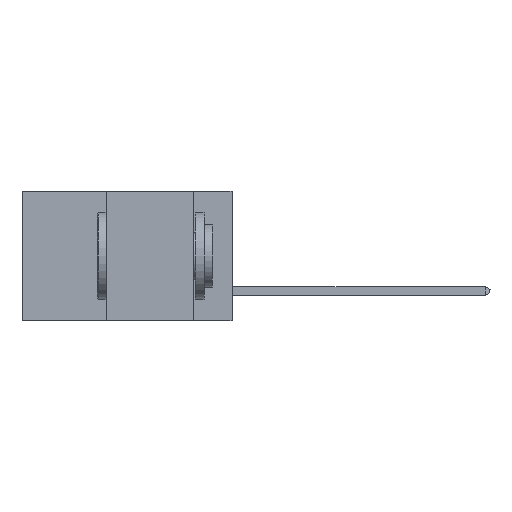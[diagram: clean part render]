
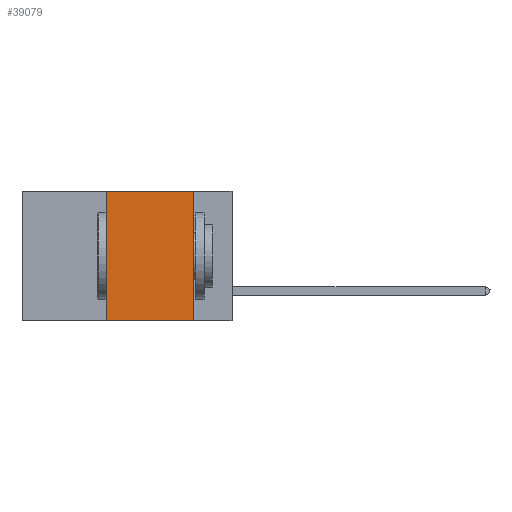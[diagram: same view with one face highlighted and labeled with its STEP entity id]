
A CAD part, left-side view. The second image highlights one B-rep face of the part: STEP entity #39079.
In plain terms, the highlighted planar face has unit normal (-1, 0, 0).
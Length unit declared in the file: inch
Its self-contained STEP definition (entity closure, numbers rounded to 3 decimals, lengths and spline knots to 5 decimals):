
#1183 = ORIENTED_EDGE ( 'NONE', *, *, #32483, .F. ) ;
#2112 = CARTESIAN_POINT ( 'NONE',  ( 0., 0.36, 0. ) ) ;
#4517 = VERTEX_POINT ( 'NONE', #10247 ) ;
#4950 = CARTESIAN_POINT ( 'NONE',  ( 0., 0.6, 0. ) ) ;
#5238 = DIRECTION ( 'NONE',  ( 1., 0., 0. ) ) ;
#6734 = EDGE_CURVE ( 'NONE', #28590, #38490, #20084, .T. ) ;
#6963 = DIRECTION ( 'NONE',  ( 0., 0., -1. ) ) ;
#7140 = VECTOR ( 'NONE', #8935, 39.37008 ) ;
#7709 = LINE ( 'NONE', #4950, #35228 ) ;
#8458 = CARTESIAN_POINT ( 'NONE',  ( 0., 0.6, 0. ) ) ;
#8526 = DIRECTION ( 'NONE',  ( 0., 0., 1. ) ) ;
#8935 = DIRECTION ( 'NONE',  ( 0., -1., 0. ) ) ;
#10247 = CARTESIAN_POINT ( 'NONE',  ( 0., 0.11, 0. ) ) ;
#12253 = CARTESIAN_POINT ( 'NONE',  ( 0., 0.6, -0.37 ) ) ;
#14355 = DIRECTION ( 'NONE',  ( 0., 0., -1. ) ) ;
#14677 = ORIENTED_EDGE ( 'NONE', *, *, #17782, .T. ) ;
#15238 = LINE ( 'NONE', #12253, #7140 ) ;
#17782 = EDGE_CURVE ( 'NONE', #28590, #37197, #15238, .T. ) ;
#18624 = VECTOR ( 'NONE', #8526, 39.37008 ) ;
#20084 = LINE ( 'NONE', #2112, #18624 ) ;
#22699 = CARTESIAN_POINT ( 'NONE',  ( 0., 0.11, 0. ) ) ;
#28173 = ORIENTED_EDGE ( 'NONE', *, *, #31020, .F. ) ;
#28590 = VERTEX_POINT ( 'NONE', #36981 ) ;
#28702 = CARTESIAN_POINT ( 'NONE',  ( 0., 0.11, -0.37 ) ) ;
#30543 = DIRECTION ( 'NONE',  ( 0., -1., 0. ) ) ;
#31020 = EDGE_CURVE ( 'NONE', #38490, #4517, #7709, .T. ) ;
#32483 = EDGE_CURVE ( 'NONE', #4517, #37197, #32607, .T. ) ;
#32607 = LINE ( 'NONE', #22699, #39689 ) ;
#32659 = CARTESIAN_POINT ( 'NONE',  ( 0., 0.36, 0. ) ) ;
#33716 = AXIS2_PLACEMENT_3D ( 'NONE', #8458, #5238, #14355 ) ;
#35228 = VECTOR ( 'NONE', #30543, 39.37008 ) ;
#36981 = CARTESIAN_POINT ( 'NONE',  ( 0., 0.36, -0.37 ) ) ;
#37197 = VERTEX_POINT ( 'NONE', #28702 ) ;
#38490 = VERTEX_POINT ( 'NONE', #32659 ) ;
#38697 = ORIENTED_EDGE ( 'NONE', *, *, #6734, .F. ) ;
#38955 = FACE_OUTER_BOUND ( 'NONE', #40923, .T. ) ;
#39079 = ADVANCED_FACE ( 'NONE', ( #38955 ), #40234, .F. ) ;
#39689 = VECTOR ( 'NONE', #6963, 39.37008 ) ;
#40234 = PLANE ( 'NONE',  #33716 ) ;
#40923 = EDGE_LOOP ( 'NONE', ( #1183, #28173, #38697, #14677 ) ) ;
